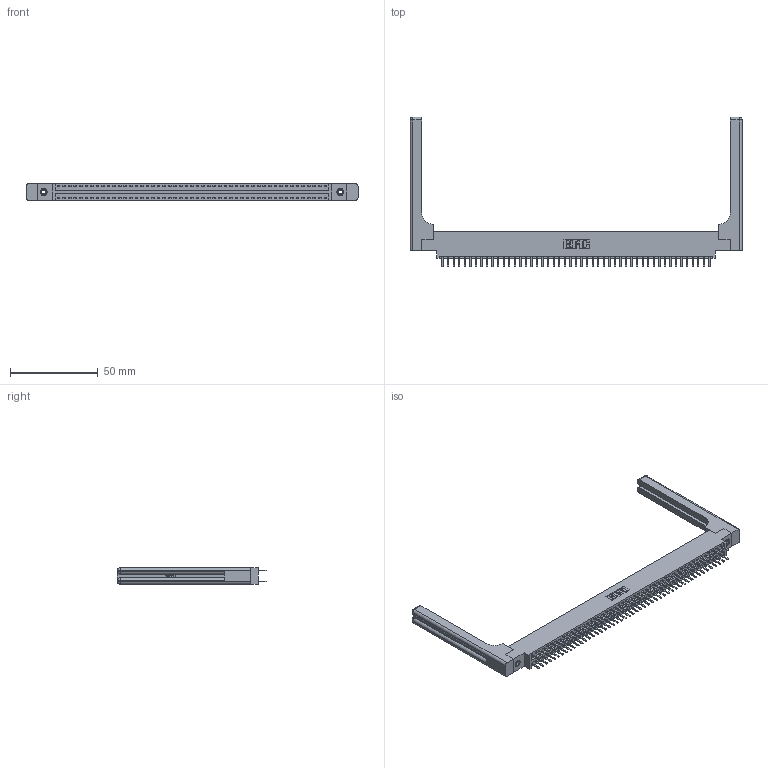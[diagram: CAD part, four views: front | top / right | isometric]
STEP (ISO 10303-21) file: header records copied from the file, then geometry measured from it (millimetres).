
FILE_DESCRIPTION (( 'STEP AP203' ), '1' );
FILE_NAME ('396-098-520-858.STEP', '2019-11-02T16:57:03', ( '' ), ( '' ), 'SwSTEP 2.0', 'SolidWorks 2016', '' );
FILE_SCHEMA (( 'CONFIG_CONTROL_DESIGN' ));
Length unit declared in the file: inch
Products named in the file (5): 345-250-001_345-250-001-102; 346-220-058_345-220-058; 396-098-520-858; 346 Part_0.170 Offset - 0.156 Dia-TH; 345-292-001_345-293-120
Assembly tree (103 placements, depth 2):
  396-098-520-858
    346 Part_0.170 Offset - 0.156 Dia-TH
    345-292-001_345-293-120  x98
    345-250-001_345-250-001-102  x2
    346-220-058_345-220-058  x2
Bounding box: 189.64 x 85.29 x 9.4 mm (x, y, z)
Volume: 25842.8 mm3; surface area: 30382.8 mm2
Topology: 103 solids, 103 shells, 5870 faces, 16981 edges, 11038 vertices
Faces by surface type: plane 3854, cylinder 1956, bspline 36, cone 12, sphere 8, torus 4
Entity records: 36464 total; most frequent: CARTESIAN_POINT 7021, ORIENTED_EDGE 5740, DIRECTION 5158, EDGE_CURVE 2870, LINE 2446, VECTOR 2446, VERTEX_POINT 1902, AXIS2_PLACEMENT_3D 1356
